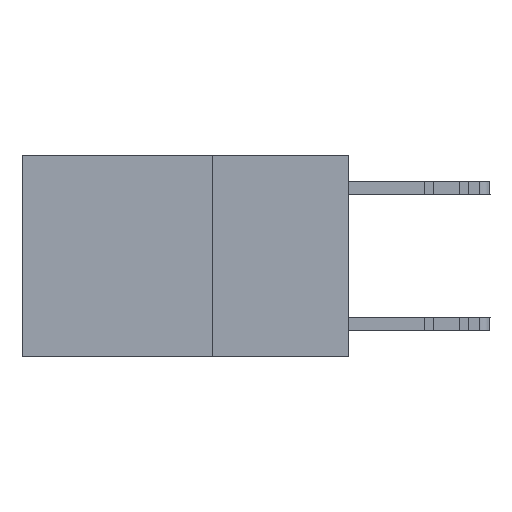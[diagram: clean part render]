
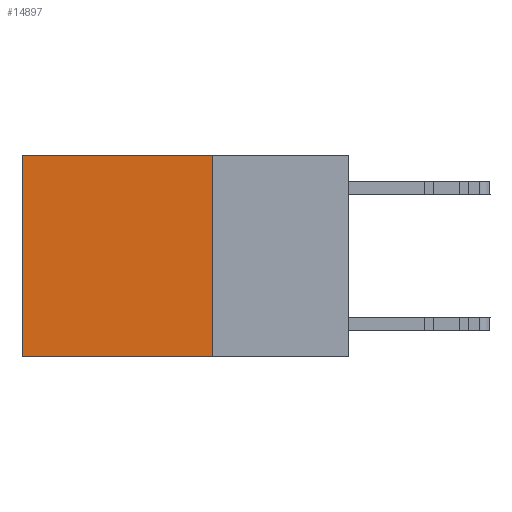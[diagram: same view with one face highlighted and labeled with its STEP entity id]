
A CAD part, left-side view. The second image highlights one B-rep face of the part: STEP entity #14897.
In plain terms, the highlighted planar face has unit normal (-1, 0, 0).
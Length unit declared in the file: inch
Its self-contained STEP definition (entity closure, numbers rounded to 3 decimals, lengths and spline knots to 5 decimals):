
#2255 = DIRECTION ( 'NONE',  ( 0., 0., -1. ) ) ;
#2291 = CARTESIAN_POINT ( 'NONE',  ( 0.2625, 0.6, 0. ) ) ;
#2374 = CARTESIAN_POINT ( 'NONE',  ( 0.2625, 0.25, -0.37 ) ) ;
#3350 = ORIENTED_EDGE ( 'NONE', *, *, #26218, .T. ) ;
#5480 = VERTEX_POINT ( 'NONE', #10480 ) ;
#7769 = ORIENTED_EDGE ( 'NONE', *, *, #20666, .F. ) ;
#8088 = AXIS2_PLACEMENT_3D ( 'NONE', #19530, #19484, #19453 ) ;
#8663 = VERTEX_POINT ( 'NONE', #21524 ) ;
#8786 = CARTESIAN_POINT ( 'NONE',  ( 0.2625, 0.25, -0.37 ) ) ;
#9148 = DIRECTION ( 'NONE',  ( 0., 1., 0. ) ) ;
#10480 = CARTESIAN_POINT ( 'NONE',  ( 0.2625, 0.25, 0. ) ) ;
#11270 = DIRECTION ( 'NONE',  ( 0., 1., 0. ) ) ;
#11859 = LINE ( 'NONE', #28087, #11911 ) ;
#11911 = VECTOR ( 'NONE', #11270, 39.37008 ) ;
#14450 = FACE_OUTER_BOUND ( 'NONE', #23645, .T. ) ;
#14897 = ADVANCED_FACE ( 'NONE', ( #14450 ), #19739, .F. ) ;
#16506 = ORIENTED_EDGE ( 'NONE', *, *, #18526, .F. ) ;
#16994 = VECTOR ( 'NONE', #2255, 39.37008 ) ;
#17954 = LINE ( 'NONE', #2291, #16994 ) ;
#18526 = EDGE_CURVE ( 'NONE', #28710, #29131, #27258, .T. ) ;
#18936 = EDGE_CURVE ( 'NONE', #8663, #29131, #17954, .T. ) ;
#19453 = DIRECTION ( 'NONE',  ( 0., 0., -1. ) ) ;
#19484 = DIRECTION ( 'NONE',  ( 1., 0., 0. ) ) ;
#19530 = CARTESIAN_POINT ( 'NONE',  ( 0.2625, 0.25, 0. ) ) ;
#19739 = PLANE ( 'NONE',  #8088 ) ;
#20666 = EDGE_CURVE ( 'NONE', #5480, #28710, #29703, .T. ) ;
#21462 = ORIENTED_EDGE ( 'NONE', *, *, #18936, .T. ) ;
#21524 = CARTESIAN_POINT ( 'NONE',  ( 0.2625, 0.6, 0. ) ) ;
#23483 = CARTESIAN_POINT ( 'NONE',  ( 0.2625, 0.6, -0.37 ) ) ;
#23645 = EDGE_LOOP ( 'NONE', ( #21462, #16506, #7769, #3350 ) ) ;
#24496 = CARTESIAN_POINT ( 'NONE',  ( 0.2625, 0.25, 0. ) ) ;
#24504 = DIRECTION ( 'NONE',  ( 0., 0., -1. ) ) ;
#26218 = EDGE_CURVE ( 'NONE', #5480, #8663, #11859, .T. ) ;
#27258 = LINE ( 'NONE', #8786, #30095 ) ;
#28087 = CARTESIAN_POINT ( 'NONE',  ( 0.2625, 0.25, 0. ) ) ;
#28710 = VERTEX_POINT ( 'NONE', #2374 ) ;
#29131 = VERTEX_POINT ( 'NONE', #23483 ) ;
#29703 = LINE ( 'NONE', #24496, #29832 ) ;
#29832 = VECTOR ( 'NONE', #24504, 39.37008 ) ;
#30095 = VECTOR ( 'NONE', #9148, 39.37008 ) ;
